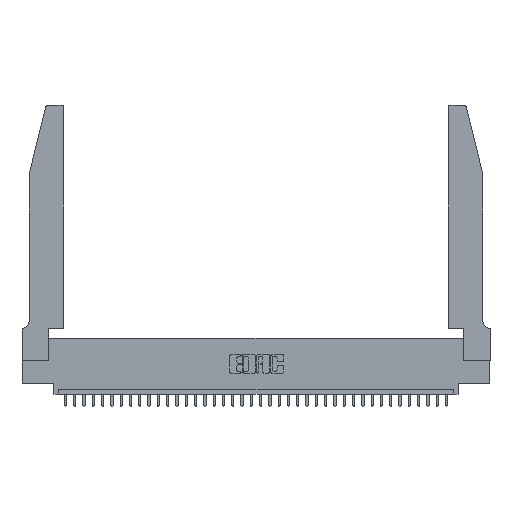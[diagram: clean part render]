
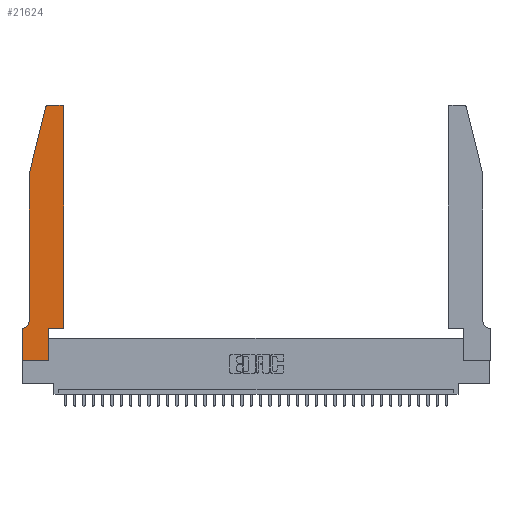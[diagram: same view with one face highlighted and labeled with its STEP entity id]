
A CAD part, top view. The second image highlights one B-rep face of the part: STEP entity #21624.
In plain terms, the highlighted planar face has unit normal (0, 0, 1).
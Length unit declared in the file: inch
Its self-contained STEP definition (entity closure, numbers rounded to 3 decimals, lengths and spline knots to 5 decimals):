
#78 = CARTESIAN_POINT ( 'NONE',  ( 0.4505, 0.35, 0.37 ) ) ;
#225 = VECTOR ( 'NONE', #1135, 39.37008 ) ;
#873 = CARTESIAN_POINT ( 'NONE',  ( 0.25487, 2.72718, 0.37 ) ) ;
#1021 = CARTESIAN_POINT ( 'NONE',  ( 0.2865, 0.35, 0.37 ) ) ;
#1091 = CARTESIAN_POINT ( 'NONE',  ( 0.4205, 2.72, 0.37 ) ) ;
#1097 = CARTESIAN_POINT ( 'NONE',  ( 0.0055, 0.35, 0.37 ) ) ;
#1135 = DIRECTION ( 'NONE',  ( 0., 1., 0. ) ) ;
#1612 = LINE ( 'NONE', #29738, #30732 ) ;
#2358 = EDGE_CURVE ( 'NONE', #11353, #7128, #4218, .T. ) ;
#2507 = CIRCLE ( 'NONE', #34968, 0.07 ) ;
#2530 = LINE ( 'NONE', #15134, #17913 ) ;
#2773 = VERTEX_POINT ( 'NONE', #14632 ) ;
#3205 = ORIENTED_EDGE ( 'NONE', *, *, #33074, .T. ) ;
#3349 = VECTOR ( 'NONE', #30725, 39.37008 ) ;
#4051 = PLANE ( 'NONE',  #18820 ) ;
#4136 = CARTESIAN_POINT ( 'NONE',  ( 0.284, 2.75, 0.37 ) ) ;
#4218 = LINE ( 'NONE', #36411, #3349 ) ;
#5189 = LINE ( 'NONE', #78, #28549 ) ;
#5318 = CARTESIAN_POINT ( 'NONE',  ( 0., 0.35, 0.37 ) ) ;
#5482 = EDGE_CURVE ( 'NONE', #20458, #21991, #30480, .T. ) ;
#6467 = DIRECTION ( 'NONE',  ( 1., 0., 0. ) ) ;
#6710 = ORIENTED_EDGE ( 'NONE', *, *, #18754, .T. ) ;
#6844 = CARTESIAN_POINT ( 'NONE',  ( 0.4505, 2.72, 0.37 ) ) ;
#6851 = EDGE_CURVE ( 'NONE', #29151, #20458, #5189, .T. ) ;
#7128 = VERTEX_POINT ( 'NONE', #5318 ) ;
#8152 = CARTESIAN_POINT ( 'NONE',  ( 0.4205, 2.75, 0.37 ) ) ;
#8278 = CARTESIAN_POINT ( 'NONE',  ( 0.2865, 0., 0.37 ) ) ;
#8599 = VERTEX_POINT ( 'NONE', #8152 ) ;
#8856 = DIRECTION ( 'NONE',  ( 0., -1., 0. ) ) ;
#8927 = DIRECTION ( 'NONE',  ( -1., 0., 0. ) ) ;
#8979 = CIRCLE ( 'NONE', #27948, 0.03 ) ;
#9152 = VECTOR ( 'NONE', #16457, 39.37008 ) ;
#11353 = VERTEX_POINT ( 'NONE', #1097 ) ;
#11526 = CARTESIAN_POINT ( 'NONE',  ( 0.0755, 2., 0.37 ) ) ;
#11542 = EDGE_CURVE ( 'NONE', #20201, #11353, #2507, .T. ) ;
#11549 = EDGE_CURVE ( 'NONE', #21991, #8599, #23156, .T. ) ;
#11806 = EDGE_CURVE ( 'NONE', #7128, #2773, #1612, .T. ) ;
#12194 = LINE ( 'NONE', #18936, #21030 ) ;
#12663 = EDGE_CURVE ( 'NONE', #14625, #29151, #15104, .T. ) ;
#13601 = CARTESIAN_POINT ( 'NONE',  ( 0.0755, 2., 0.37 ) ) ;
#14625 = VERTEX_POINT ( 'NONE', #8278 ) ;
#14632 = CARTESIAN_POINT ( 'NONE',  ( 0., 0., 0.37 ) ) ;
#14844 = DIRECTION ( 'NONE',  ( 1., 0., 0. ) ) ;
#15104 = LINE ( 'NONE', #1021, #225 ) ;
#15134 = CARTESIAN_POINT ( 'NONE',  ( 0., 0., 0.37 ) ) ;
#15336 = ORIENTED_EDGE ( 'NONE', *, *, #12663, .T. ) ;
#15477 = CARTESIAN_POINT ( 'NONE',  ( 0.0755, 0.42, 0.37 ) ) ;
#15563 = DIRECTION ( 'NONE',  ( 0., 0., 1. ) ) ;
#15741 = ORIENTED_EDGE ( 'NONE', *, *, #11549, .T. ) ;
#16455 = CARTESIAN_POINT ( 'NONE',  ( 0.284, 2.72, 0.37 ) ) ;
#16457 = DIRECTION ( 'NONE',  ( -0.239, -0.971, 0. ) ) ;
#16538 = LINE ( 'NONE', #11526, #34279 ) ;
#16869 = ORIENTED_EDGE ( 'NONE', *, *, #5482, .T. ) ;
#17127 = ORIENTED_EDGE ( 'NONE', *, *, #11806, .T. ) ;
#17287 = CARTESIAN_POINT ( 'NONE',  ( 0.0755, 2., 0.37 ) ) ;
#17421 = EDGE_CURVE ( 'NONE', #36150, #32943, #35663, .T. ) ;
#17543 = ORIENTED_EDGE ( 'NONE', *, *, #2358, .T. ) ;
#17650 = FACE_OUTER_BOUND ( 'NONE', #29996, .T. ) ;
#17913 = VECTOR ( 'NONE', #6467, 39.37008 ) ;
#17996 = DIRECTION ( 'NONE',  ( 0., -1., 0. ) ) ;
#18754 = EDGE_CURVE ( 'NONE', #32943, #20201, #16538, .T. ) ;
#18820 = AXIS2_PLACEMENT_3D ( 'NONE', #24113, #15563, #23857 ) ;
#18936 = CARTESIAN_POINT ( 'NONE',  ( 0.2605, 2.75, 0.37 ) ) ;
#19307 = DIRECTION ( 'NONE',  ( 1., 0., 0. ) ) ;
#20201 = VERTEX_POINT ( 'NONE', #15477 ) ;
#20458 = VERTEX_POINT ( 'NONE', #21775 ) ;
#21030 = VECTOR ( 'NONE', #35640, 39.37008 ) ;
#21058 = ORIENTED_EDGE ( 'NONE', *, *, #34134, .T. ) ;
#21226 = DIRECTION ( 'NONE',  ( 0., 1., 0. ) ) ;
#21295 = CARTESIAN_POINT ( 'NONE',  ( 0.2865, 0.35, 0.37 ) ) ;
#21624 = ADVANCED_FACE ( 'NONE', ( #17650 ), #4051, .T. ) ;
#21775 = CARTESIAN_POINT ( 'NONE',  ( 0.4505, 0.35, 0.37 ) ) ;
#21923 = DIRECTION ( 'NONE',  ( 1., 0., 0. ) ) ;
#21991 = VERTEX_POINT ( 'NONE', #6844 ) ;
#22763 = ORIENTED_EDGE ( 'NONE', *, *, #17421, .T. ) ;
#23156 = CIRCLE ( 'NONE', #34285, 0.03 ) ;
#23857 = DIRECTION ( 'NONE',  ( 1., 0., 0. ) ) ;
#24113 = CARTESIAN_POINT ( 'NONE',  ( 0., 0.35, 0.37 ) ) ;
#25965 = DIRECTION ( 'NONE',  ( 0., 0., -1. ) ) ;
#27010 = ORIENTED_EDGE ( 'NONE', *, *, #6851, .T. ) ;
#27910 = EDGE_CURVE ( 'NONE', #8599, #34438, #12194, .T. ) ;
#27948 = AXIS2_PLACEMENT_3D ( 'NONE', #16455, #36258, #19307 ) ;
#28549 = VECTOR ( 'NONE', #21923, 39.37008 ) ;
#29151 = VERTEX_POINT ( 'NONE', #21295 ) ;
#29738 = CARTESIAN_POINT ( 'NONE',  ( 0., 0., 0.37 ) ) ;
#29996 = EDGE_LOOP ( 'NONE', ( #34788, #21058, #22763, #6710, #33248, #17543, #17127, #3205, #15336, #27010, #16869, #15741 ) ) ;
#30480 = LINE ( 'NONE', #32237, #33149 ) ;
#30725 = DIRECTION ( 'NONE',  ( -1., 0., 0. ) ) ;
#30732 = VECTOR ( 'NONE', #17996, 39.37008 ) ;
#32237 = CARTESIAN_POINT ( 'NONE',  ( 0.4505, 0.35, 0.37 ) ) ;
#32943 = VERTEX_POINT ( 'NONE', #17287 ) ;
#33074 = EDGE_CURVE ( 'NONE', #2773, #14625, #2530, .T. ) ;
#33149 = VECTOR ( 'NONE', #21226, 39.37008 ) ;
#33248 = ORIENTED_EDGE ( 'NONE', *, *, #11542, .T. ) ;
#34134 = EDGE_CURVE ( 'NONE', #34438, #36150, #8979, .T. ) ;
#34279 = VECTOR ( 'NONE', #8856, 39.37008 ) ;
#34285 = AXIS2_PLACEMENT_3D ( 'NONE', #1091, #34749, #14844 ) ;
#34438 = VERTEX_POINT ( 'NONE', #4136 ) ;
#34510 = CARTESIAN_POINT ( 'NONE',  ( 0.0055, 0.42, 0.37 ) ) ;
#34749 = DIRECTION ( 'NONE',  ( 0., 0., 1. ) ) ;
#34788 = ORIENTED_EDGE ( 'NONE', *, *, #27910, .T. ) ;
#34968 = AXIS2_PLACEMENT_3D ( 'NONE', #34510, #25965, #8927 ) ;
#35640 = DIRECTION ( 'NONE',  ( -1., 0., 0. ) ) ;
#35663 = LINE ( 'NONE', #13601, #9152 ) ;
#36150 = VERTEX_POINT ( 'NONE', #873 ) ;
#36258 = DIRECTION ( 'NONE',  ( 0., 0., 1. ) ) ;
#36411 = CARTESIAN_POINT ( 'NONE',  ( 0.0755, 0.35, 0.37 ) ) ;
